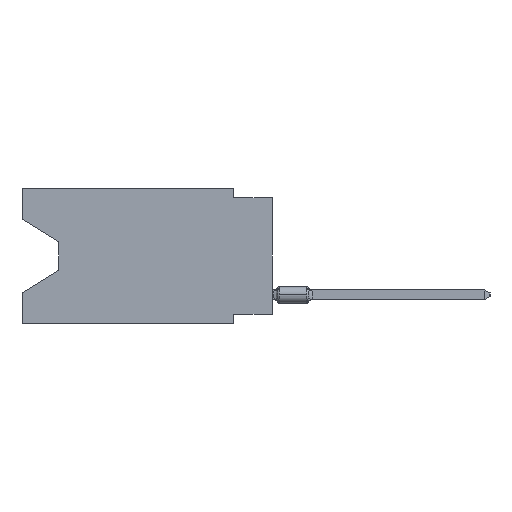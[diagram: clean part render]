
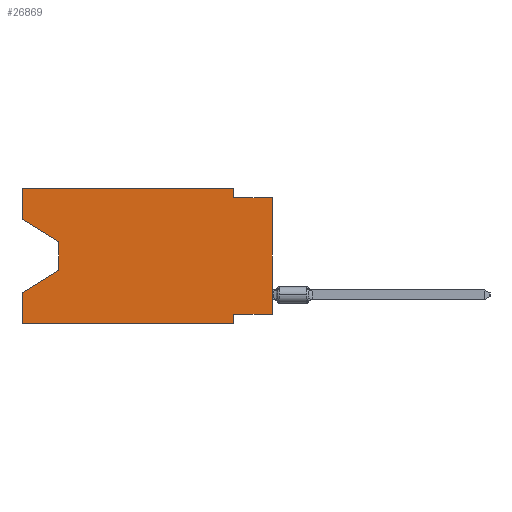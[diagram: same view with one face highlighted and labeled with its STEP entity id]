
A CAD part, left-side view. The second image highlights one B-rep face of the part: STEP entity #26869.
In plain terms, the highlighted planar face has unit normal (-1, 0, 0).
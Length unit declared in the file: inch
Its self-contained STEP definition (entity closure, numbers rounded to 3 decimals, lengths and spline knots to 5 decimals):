
#141 = VERTEX_POINT ( 'NONE', #30646 ) ;
#476 = LINE ( 'NONE', #32333, #39797 ) ;
#1233 = DIRECTION ( 'NONE',  ( 0., 0., -1. ) ) ;
#1659 = CARTESIAN_POINT ( 'NONE',  ( 0., 0., -0.025 ) ) ;
#2394 = ORIENTED_EDGE ( 'NONE', *, *, #13684, .F. ) ;
#2403 = DIRECTION ( 'NONE',  ( 0., -0.855, -0.519 ) ) ;
#3827 = CARTESIAN_POINT ( 'NONE',  ( 0., 0.645, 0. ) ) ;
#4028 = EDGE_CURVE ( 'NONE', #9277, #16921, #32416, .T. ) ;
#4458 = CARTESIAN_POINT ( 'NONE',  ( 0., 0.55, -0.138 ) ) ;
#5392 = CARTESIAN_POINT ( 'NONE',  ( 0., 0., -0.025 ) ) ;
#5447 = EDGE_CURVE ( 'NONE', #17665, #23387, #41017, .T. ) ;
#6038 = CARTESIAN_POINT ( 'NONE',  ( 0., 0., -0.325 ) ) ;
#6295 = ORIENTED_EDGE ( 'NONE', *, *, #16341, .F. ) ;
#7378 = VERTEX_POINT ( 'NONE', #20509 ) ;
#7411 = VERTEX_POINT ( 'NONE', #27492 ) ;
#8158 = VECTOR ( 'NONE', #14760, 39.37008 ) ;
#8186 = LINE ( 'NONE', #29115, #36295 ) ;
#9277 = VERTEX_POINT ( 'NONE', #9367 ) ;
#9367 = CARTESIAN_POINT ( 'NONE',  ( 0., 0.645, -0.35 ) ) ;
#9379 = PLANE ( 'NONE',  #33272 ) ;
#9906 = CARTESIAN_POINT ( 'NONE',  ( 0., 0.1, -0.325 ) ) ;
#11888 = LINE ( 'NONE', #4458, #25278 ) ;
#11916 = LINE ( 'NONE', #5392, #24979 ) ;
#12666 = ORIENTED_EDGE ( 'NONE', *, *, #35788, .T. ) ;
#13684 = EDGE_CURVE ( 'NONE', #23387, #17753, #33637, .T. ) ;
#13757 = DIRECTION ( 'NONE',  ( 0., 0.855, -0.519 ) ) ;
#14488 = CARTESIAN_POINT ( 'NONE',  ( 0., 0.645, -0.35 ) ) ;
#14760 = DIRECTION ( 'NONE',  ( 0., 0., 1. ) ) ;
#15052 = DIRECTION ( 'NONE',  ( 0., 0., -1. ) ) ;
#15554 = VECTOR ( 'NONE', #17625, 39.37008 ) ;
#15852 = CARTESIAN_POINT ( 'NONE',  ( 0., 0.645, 0. ) ) ;
#16086 = CARTESIAN_POINT ( 'NONE',  ( 0., 0.1, -0.025 ) ) ;
#16260 = CARTESIAN_POINT ( 'NONE',  ( 0., 0.645, -0.26975 ) ) ;
#16341 = EDGE_CURVE ( 'NONE', #141, #17665, #8186, .T. ) ;
#16799 = CARTESIAN_POINT ( 'NONE',  ( 0., 0.645, 0. ) ) ;
#16921 = VERTEX_POINT ( 'NONE', #16260 ) ;
#16986 = EDGE_CURVE ( 'NONE', #30694, #37681, #42489, .T. ) ;
#17148 = VECTOR ( 'NONE', #42846, 39.37008 ) ;
#17611 = VERTEX_POINT ( 'NONE', #1659 ) ;
#17625 = DIRECTION ( 'NONE',  ( 0., 1., 0. ) ) ;
#17665 = VERTEX_POINT ( 'NONE', #15852 ) ;
#17753 = VERTEX_POINT ( 'NONE', #16086 ) ;
#20509 = CARTESIAN_POINT ( 'NONE',  ( 0., 0.55, -0.138 ) ) ;
#20541 = CARTESIAN_POINT ( 'NONE',  ( 0., 0.645, -0.08025 ) ) ;
#20603 = VECTOR ( 'NONE', #40319, 39.37008 ) ;
#20903 = ORIENTED_EDGE ( 'NONE', *, *, #45800, .T. ) ;
#21065 = VECTOR ( 'NONE', #15052, 39.37008 ) ;
#21777 = ORIENTED_EDGE ( 'NONE', *, *, #45870, .F. ) ;
#23387 = VERTEX_POINT ( 'NONE', #35349 ) ;
#23875 = LINE ( 'NONE', #35476, #24523 ) ;
#24383 = CARTESIAN_POINT ( 'NONE',  ( 0., 0., -0.325 ) ) ;
#24523 = VECTOR ( 'NONE', #28267, 39.37008 ) ;
#24979 = VECTOR ( 'NONE', #33528, 39.37008 ) ;
#25278 = VECTOR ( 'NONE', #39785, 39.37008 ) ;
#25283 = ORIENTED_EDGE ( 'NONE', *, *, #25606, .T. ) ;
#25606 = EDGE_CURVE ( 'NONE', #7411, #16921, #476, .T. ) ;
#25656 = CARTESIAN_POINT ( 'NONE',  ( 0., 0.1, -0.35 ) ) ;
#26869 = ADVANCED_FACE ( 'NONE', ( #41225 ), #9379, .F. ) ;
#27492 = CARTESIAN_POINT ( 'NONE',  ( 0., 0.55, -0.212 ) ) ;
#27498 = ORIENTED_EDGE ( 'NONE', *, *, #31468, .T. ) ;
#27989 = VECTOR ( 'NONE', #2403, 39.37008 ) ;
#28267 = DIRECTION ( 'NONE',  ( 0., 0., 1. ) ) ;
#28932 = CARTESIAN_POINT ( 'NONE',  ( 0., 0.1, -0.35 ) ) ;
#29115 = CARTESIAN_POINT ( 'NONE',  ( 0., 0.645, 0. ) ) ;
#29387 = LINE ( 'NONE', #28932, #44012 ) ;
#29919 = CARTESIAN_POINT ( 'NONE',  ( 0., 0.1, 0. ) ) ;
#30646 = CARTESIAN_POINT ( 'NONE',  ( 0., 0.645, -0.08025 ) ) ;
#30694 = VERTEX_POINT ( 'NONE', #6038 ) ;
#31468 = EDGE_CURVE ( 'NONE', #30694, #17611, #23875, .T. ) ;
#32145 = LINE ( 'NONE', #14488, #17148 ) ;
#32333 = CARTESIAN_POINT ( 'NONE',  ( 0., 0.55, -0.212 ) ) ;
#32416 = LINE ( 'NONE', #3827, #8158 ) ;
#33272 = AXIS2_PLACEMENT_3D ( 'NONE', #16799, #45160, #42568 ) ;
#33456 = ORIENTED_EDGE ( 'NONE', *, *, #42492, .F. ) ;
#33528 = DIRECTION ( 'NONE',  ( 0., -1., 0. ) ) ;
#33637 = LINE ( 'NONE', #29919, #21065 ) ;
#34260 = LINE ( 'NONE', #20541, #27989 ) ;
#34650 = ORIENTED_EDGE ( 'NONE', *, *, #4028, .F. ) ;
#35349 = CARTESIAN_POINT ( 'NONE',  ( 0., 0.1, 0. ) ) ;
#35476 = CARTESIAN_POINT ( 'NONE',  ( 0., 0., 0. ) ) ;
#35788 = EDGE_CURVE ( 'NONE', #141, #7378, #34260, .T. ) ;
#36295 = VECTOR ( 'NONE', #43061, 39.37008 ) ;
#37681 = VERTEX_POINT ( 'NONE', #9906 ) ;
#38897 = ORIENTED_EDGE ( 'NONE', *, *, #5447, .F. ) ;
#39785 = DIRECTION ( 'NONE',  ( 0., 0., -1. ) ) ;
#39797 = VECTOR ( 'NONE', #13757, 39.37008 ) ;
#39819 = EDGE_CURVE ( 'NONE', #7378, #7411, #11888, .T. ) ;
#39944 = EDGE_LOOP ( 'NONE', ( #12666, #41482, #25283, #34650, #20903, #33456, #45370, #27498, #21777, #2394, #38897, #6295 ) ) ;
#40319 = DIRECTION ( 'NONE',  ( 0., -1., 0. ) ) ;
#41017 = LINE ( 'NONE', #43809, #20603 ) ;
#41225 = FACE_OUTER_BOUND ( 'NONE', #39944, .T. ) ;
#41329 = VERTEX_POINT ( 'NONE', #25656 ) ;
#41482 = ORIENTED_EDGE ( 'NONE', *, *, #39819, .T. ) ;
#42489 = LINE ( 'NONE', #24383, #15554 ) ;
#42492 = EDGE_CURVE ( 'NONE', #37681, #41329, #29387, .T. ) ;
#42568 = DIRECTION ( 'NONE',  ( 0., 0., -1. ) ) ;
#42846 = DIRECTION ( 'NONE',  ( 0., -1., 0. ) ) ;
#43061 = DIRECTION ( 'NONE',  ( 0., 0., 1. ) ) ;
#43809 = CARTESIAN_POINT ( 'NONE',  ( 0., 0.645, 0. ) ) ;
#44012 = VECTOR ( 'NONE', #1233, 39.37008 ) ;
#45160 = DIRECTION ( 'NONE',  ( 1., 0., 0. ) ) ;
#45370 = ORIENTED_EDGE ( 'NONE', *, *, #16986, .F. ) ;
#45800 = EDGE_CURVE ( 'NONE', #9277, #41329, #32145, .T. ) ;
#45870 = EDGE_CURVE ( 'NONE', #17753, #17611, #11916, .T. ) ;
